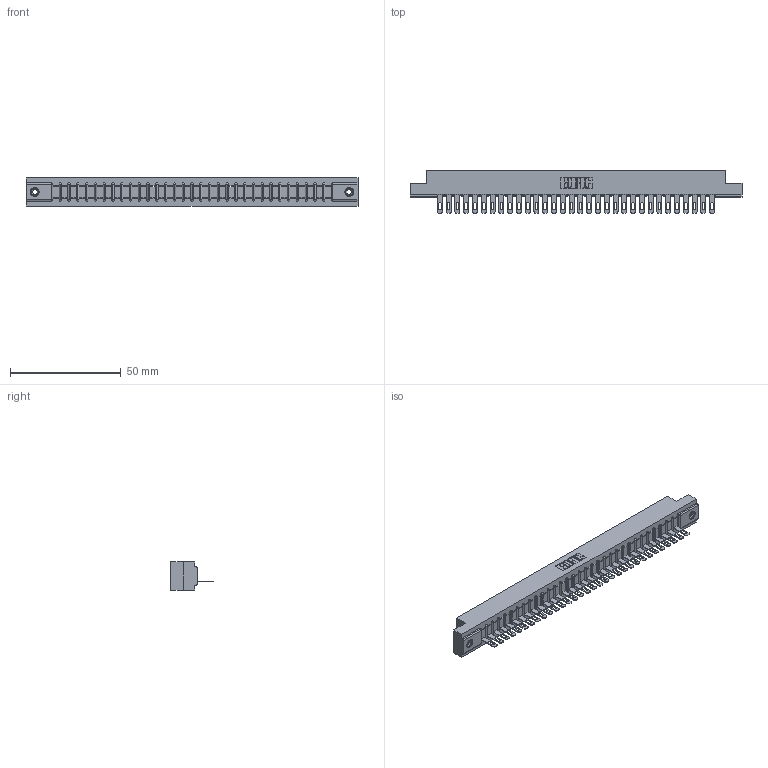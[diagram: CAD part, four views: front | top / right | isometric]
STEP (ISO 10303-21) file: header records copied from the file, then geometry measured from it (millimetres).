
FILE_DESCRIPTION (( 'STEP AP203' ), '1' );
FILE_NAME ('357-032-405-108.STEP', '2020-10-02T04:25:07', ( '' ), ( '' ), 'SwSTEP 2.0', 'SolidWorks 2020', '' );
FILE_SCHEMA (( 'CONFIG_CONTROL_DESIGN' ));
Length unit declared in the file: inch
Products named in the file (4): 307-290-001_505; 345-250-001_345-250-003-102; 307 Part_.156 Dia Mounting Holes; 357-032-405-108
Assembly tree (35 placements, depth 2):
  357-032-405-108
    307 Part_.156 Dia Mounting Holes
    307-290-001_505  x32
    345-250-001_345-250-003-102  x2
Bounding box: 149.81 x 19.18 x 12.7 mm (x, y, z)
Volume: 15531.9 mm3; surface area: 16621.8 mm2
Topology: 35 solids, 35 shells, 2003 faces, 5643 edges, 3622 vertices
Faces by surface type: plane 1254, cylinder 667, sphere 66, cone 12, torus 4
Entity records: 29825 total; most frequent: CARTESIAN_POINT 4999, ORIENTED_EDGE 4978, DIRECTION 4879, EDGE_CURVE 2489, LINE 1903, VECTOR 1903, VERTEX_POINT 1608, AXIS2_PLACEMENT_3D 1488
